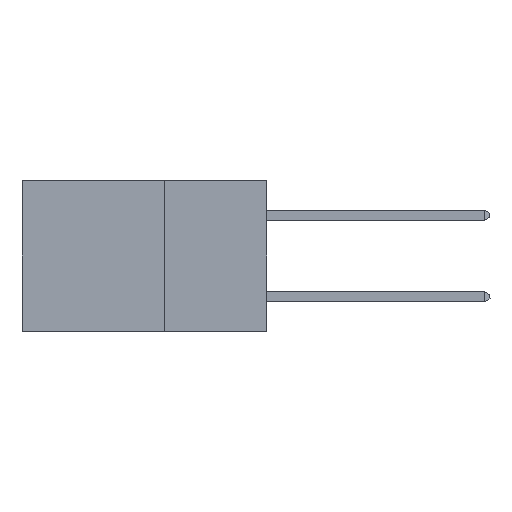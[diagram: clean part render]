
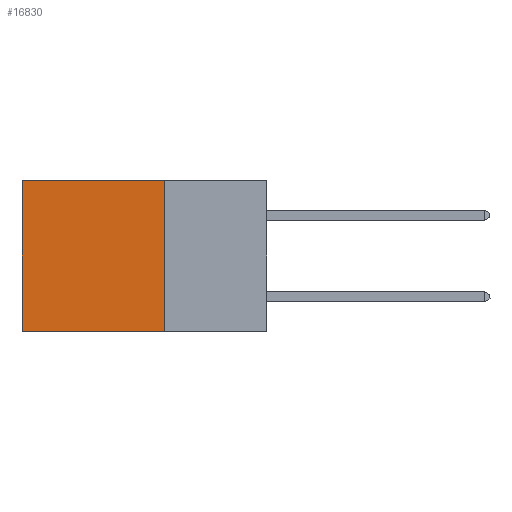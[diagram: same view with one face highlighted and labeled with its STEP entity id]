
A CAD part, left-side view. The second image highlights one B-rep face of the part: STEP entity #16830.
In plain terms, the highlighted planar face has unit normal (-1, 0, 0).
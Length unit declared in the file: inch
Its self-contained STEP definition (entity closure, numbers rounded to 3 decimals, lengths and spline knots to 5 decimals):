
#291 = CARTESIAN_POINT ( 'NONE',  ( 0.2875, 0.25, 0. ) ) ;
#1766 = VERTEX_POINT ( 'NONE', #11583 ) ;
#2808 = CARTESIAN_POINT ( 'NONE',  ( 0.2875, 0.6, 0. ) ) ;
#4687 = ORIENTED_EDGE ( 'NONE', *, *, #12668, .T. ) ;
#5470 = LINE ( 'NONE', #2808, #14872 ) ;
#6171 = CARTESIAN_POINT ( 'NONE',  ( 0.2875, 0.6, 0. ) ) ;
#7543 = VECTOR ( 'NONE', #20280, 39.37008 ) ;
#9172 = LINE ( 'NONE', #291, #16797 ) ;
#9608 = EDGE_CURVE ( 'NONE', #16915, #1766, #16361, .T. ) ;
#9708 = CARTESIAN_POINT ( 'NONE',  ( 0.2875, 0.25, -0.37 ) ) ;
#9978 = PLANE ( 'NONE',  #14774 ) ;
#10404 = ORIENTED_EDGE ( 'NONE', *, *, #21093, .F. ) ;
#10444 = CARTESIAN_POINT ( 'NONE',  ( 0.2875, 0.25, 0. ) ) ;
#11291 = VERTEX_POINT ( 'NONE', #6171 ) ;
#11583 = CARTESIAN_POINT ( 'NONE',  ( 0.2875, 0.6, -0.37 ) ) ;
#11646 = ORIENTED_EDGE ( 'NONE', *, *, #9608, .F. ) ;
#11781 = DIRECTION ( 'NONE',  ( 0., 0., -1. ) ) ;
#12668 = EDGE_CURVE ( 'NONE', #11291, #1766, #5470, .T. ) ;
#12805 = VECTOR ( 'NONE', #22958, 39.37008 ) ;
#13335 = LINE ( 'NONE', #21166, #12805 ) ;
#14471 = DIRECTION ( 'NONE',  ( 0., 0., -1. ) ) ;
#14774 = AXIS2_PLACEMENT_3D ( 'NONE', #16875, #22351, #11781 ) ;
#14872 = VECTOR ( 'NONE', #15165, 39.37008 ) ;
#15165 = DIRECTION ( 'NONE',  ( 0., 0., -1. ) ) ;
#16361 = LINE ( 'NONE', #9708, #7543 ) ;
#16797 = VECTOR ( 'NONE', #14471, 39.37008 ) ;
#16830 = ADVANCED_FACE ( 'NONE', ( #18318 ), #9978, .F. ) ;
#16866 = ORIENTED_EDGE ( 'NONE', *, *, #18857, .T. ) ;
#16875 = CARTESIAN_POINT ( 'NONE',  ( 0.2875, 0.25, 0. ) ) ;
#16915 = VERTEX_POINT ( 'NONE', #20768 ) ;
#18318 = FACE_OUTER_BOUND ( 'NONE', #21516, .T. ) ;
#18857 = EDGE_CURVE ( 'NONE', #22496, #11291, #13335, .T. ) ;
#20280 = DIRECTION ( 'NONE',  ( 0., 1., 0. ) ) ;
#20768 = CARTESIAN_POINT ( 'NONE',  ( 0.2875, 0.25, -0.37 ) ) ;
#21093 = EDGE_CURVE ( 'NONE', #22496, #16915, #9172, .T. ) ;
#21166 = CARTESIAN_POINT ( 'NONE',  ( 0.2875, 0.25, 0. ) ) ;
#21516 = EDGE_LOOP ( 'NONE', ( #4687, #11646, #10404, #16866 ) ) ;
#22351 = DIRECTION ( 'NONE',  ( 1., 0., 0. ) ) ;
#22496 = VERTEX_POINT ( 'NONE', #10444 ) ;
#22958 = DIRECTION ( 'NONE',  ( 0., 1., 0. ) ) ;
